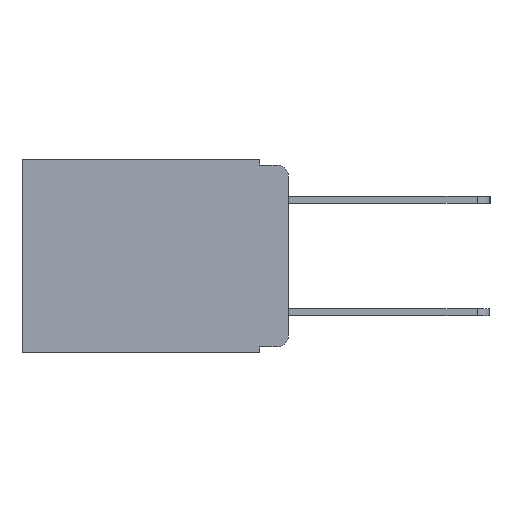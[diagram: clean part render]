
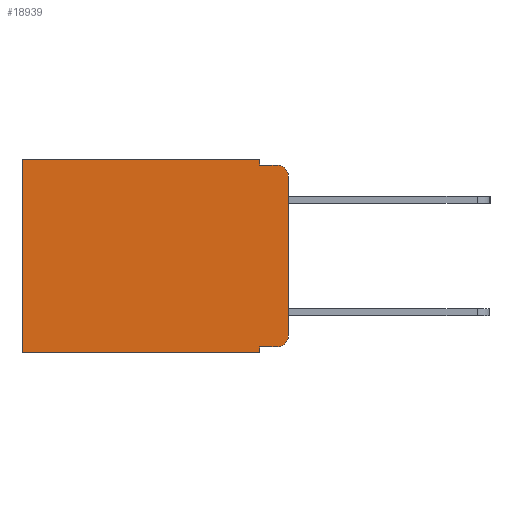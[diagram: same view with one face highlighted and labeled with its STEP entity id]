
A CAD part, left-side view. The second image highlights one B-rep face of the part: STEP entity #18939.
In plain terms, the highlighted planar face has unit normal (-1, 0, 0).
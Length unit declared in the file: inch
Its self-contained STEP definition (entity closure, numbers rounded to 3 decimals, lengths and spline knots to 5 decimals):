
#354 = ORIENTED_EDGE ( 'NONE', *, *, #1111, .T. ) ;
#458 = DIRECTION ( 'NONE',  ( 1., 0., 0. ) ) ;
#603 = EDGE_CURVE ( 'NONE', #1220, #2550, #18932, .T. ) ;
#616 = LINE ( 'NONE', #11983, #4792 ) ;
#619 = VERTEX_POINT ( 'NONE', #3339 ) ;
#671 = DIRECTION ( 'NONE',  ( 0., 1., 0. ) ) ;
#1111 = EDGE_CURVE ( 'NONE', #14233, #14268, #17338, .T. ) ;
#1220 = VERTEX_POINT ( 'NONE', #12869 ) ;
#2263 = VECTOR ( 'NONE', #3954, 39.37008 ) ;
#2452 = ORIENTED_EDGE ( 'NONE', *, *, #603, .F. ) ;
#2503 = VECTOR ( 'NONE', #6673, 39.37008 ) ;
#2520 = LINE ( 'NONE', #3759, #13689 ) ;
#2550 = VERTEX_POINT ( 'NONE', #13246 ) ;
#2767 = CARTESIAN_POINT ( 'NONE',  ( 0.298, 0.02, -0.333 ) ) ;
#2961 = DIRECTION ( 'NONE',  ( -1., 0., 0. ) ) ;
#3065 = EDGE_CURVE ( 'NONE', #2550, #13795, #2520, .T. ) ;
#3339 = CARTESIAN_POINT ( 'NONE',  ( 0.298, 0.473, 0. ) ) ;
#3467 = EDGE_LOOP ( 'NONE', ( #17980, #7461, #19345, #2452, #19155, #9657, #4435, #19945, #10921, #354 ) ) ;
#3507 = EDGE_CURVE ( 'NONE', #4394, #14233, #15145, .T. ) ;
#3759 = CARTESIAN_POINT ( 'NONE',  ( 0.298, 0.051, -0.01 ) ) ;
#3954 = DIRECTION ( 'NONE',  ( 0., 1., 0. ) ) ;
#4039 = PLANE ( 'NONE',  #15009 ) ;
#4225 = DIRECTION ( 'NONE',  ( 0., 0., -1. ) ) ;
#4236 = EDGE_CURVE ( 'NONE', #8261, #13795, #10713, .T. ) ;
#4394 = VERTEX_POINT ( 'NONE', #15193 ) ;
#4435 = ORIENTED_EDGE ( 'NONE', *, *, #10806, .F. ) ;
#4753 = VERTEX_POINT ( 'NONE', #8619 ) ;
#4792 = VECTOR ( 'NONE', #10524, 39.37008 ) ;
#5190 = CARTESIAN_POINT ( 'NONE',  ( 0.298, 0.051, -0.333 ) ) ;
#5538 = DIRECTION ( 'NONE',  ( -1., 0., 0. ) ) ;
#5550 = DIRECTION ( 'NONE',  ( 0., 0., -1. ) ) ;
#5565 = DIRECTION ( 'NONE',  ( 0., 0., -1. ) ) ;
#5579 = CARTESIAN_POINT ( 'NONE',  ( 0.298, 0., 0. ) ) ;
#5970 = CARTESIAN_POINT ( 'NONE',  ( 0.298, 0.02, -0.313 ) ) ;
#6673 = DIRECTION ( 'NONE',  ( 0., -1., 0. ) ) ;
#6896 = LINE ( 'NONE', #7559, #14691 ) ;
#6922 = FACE_OUTER_BOUND ( 'NONE', #3467, .T. ) ;
#7439 = EDGE_CURVE ( 'NONE', #8261, #14268, #616, .T. ) ;
#7461 = ORIENTED_EDGE ( 'NONE', *, *, #4236, .T. ) ;
#7559 = CARTESIAN_POINT ( 'NONE',  ( 0.298, 0., -0.343 ) ) ;
#8012 = CARTESIAN_POINT ( 'NONE',  ( 0.298, 0.051, 0. ) ) ;
#8261 = VERTEX_POINT ( 'NONE', #13556 ) ;
#8413 = AXIS2_PLACEMENT_3D ( 'NONE', #5970, #5538, #5565 ) ;
#8424 = DIRECTION ( 'NONE',  ( 0., 0., -1. ) ) ;
#8474 = DIRECTION ( 'NONE',  ( 0., -1., 0. ) ) ;
#8619 = CARTESIAN_POINT ( 'NONE',  ( 0.298, 0.473, -0.343 ) ) ;
#8953 = CARTESIAN_POINT ( 'NONE',  ( 0.298, 0.473, 0. ) ) ;
#9275 = CARTESIAN_POINT ( 'NONE',  ( 0.298, 0.02, -0.03 ) ) ;
#9657 = ORIENTED_EDGE ( 'NONE', *, *, #18078, .T. ) ;
#9840 = VERTEX_POINT ( 'NONE', #14998 ) ;
#10122 = CARTESIAN_POINT ( 'NONE',  ( 0.298, 0., -0.313 ) ) ;
#10369 = CARTESIAN_POINT ( 'NONE',  ( 0.298, 0., 0. ) ) ;
#10524 = DIRECTION ( 'NONE',  ( 0., 0., -1. ) ) ;
#10713 = CIRCLE ( 'NONE', #14304, 0.02 ) ;
#10806 = EDGE_CURVE ( 'NONE', #9840, #4753, #6896, .T. ) ;
#10855 = VECTOR ( 'NONE', #8424, 39.37008 ) ;
#10921 = ORIENTED_EDGE ( 'NONE', *, *, #3507, .T. ) ;
#11643 = CARTESIAN_POINT ( 'NONE',  ( 0.298, 0.02, -0.01 ) ) ;
#11790 = LINE ( 'NONE', #8953, #20295 ) ;
#11896 = DIRECTION ( 'NONE',  ( 0., 0., -1. ) ) ;
#11983 = CARTESIAN_POINT ( 'NONE',  ( 0.298, 0., 0. ) ) ;
#12869 = CARTESIAN_POINT ( 'NONE',  ( 0.298, 0.051, 0. ) ) ;
#13246 = CARTESIAN_POINT ( 'NONE',  ( 0.298, 0.051, -0.01 ) ) ;
#13537 = CARTESIAN_POINT ( 'NONE',  ( 0.298, 0.051, 0. ) ) ;
#13556 = CARTESIAN_POINT ( 'NONE',  ( 0.298, 0., -0.03 ) ) ;
#13689 = VECTOR ( 'NONE', #8474, 39.37008 ) ;
#13795 = VERTEX_POINT ( 'NONE', #11643 ) ;
#14233 = VERTEX_POINT ( 'NONE', #2767 ) ;
#14268 = VERTEX_POINT ( 'NONE', #10122 ) ;
#14304 = AXIS2_PLACEMENT_3D ( 'NONE', #9275, #2961, #5550 ) ;
#14691 = VECTOR ( 'NONE', #671, 39.37008 ) ;
#14926 = LINE ( 'NONE', #5579, #2263 ) ;
#14998 = CARTESIAN_POINT ( 'NONE',  ( 0.298, 0.051, -0.343 ) ) ;
#15009 = AXIS2_PLACEMENT_3D ( 'NONE', #10369, #458, #11896 ) ;
#15033 = EDGE_CURVE ( 'NONE', #1220, #619, #14926, .T. ) ;
#15145 = LINE ( 'NONE', #5190, #2503 ) ;
#15193 = CARTESIAN_POINT ( 'NONE',  ( 0.298, 0.051, -0.333 ) ) ;
#15797 = LINE ( 'NONE', #13537, #19192 ) ;
#17120 = EDGE_CURVE ( 'NONE', #4394, #9840, #15797, .T. ) ;
#17338 = CIRCLE ( 'NONE', #8413, 0.02 ) ;
#17980 = ORIENTED_EDGE ( 'NONE', *, *, #7439, .F. ) ;
#18078 = EDGE_CURVE ( 'NONE', #619, #4753, #11790, .T. ) ;
#18932 = LINE ( 'NONE', #8012, #10855 ) ;
#18939 = ADVANCED_FACE ( 'NONE', ( #6922 ), #4039, .F. ) ;
#19155 = ORIENTED_EDGE ( 'NONE', *, *, #15033, .T. ) ;
#19192 = VECTOR ( 'NONE', #4225, 39.37008 ) ;
#19345 = ORIENTED_EDGE ( 'NONE', *, *, #3065, .F. ) ;
#19565 = DIRECTION ( 'NONE',  ( 0., 0., -1. ) ) ;
#19945 = ORIENTED_EDGE ( 'NONE', *, *, #17120, .F. ) ;
#20295 = VECTOR ( 'NONE', #19565, 39.37008 ) ;
